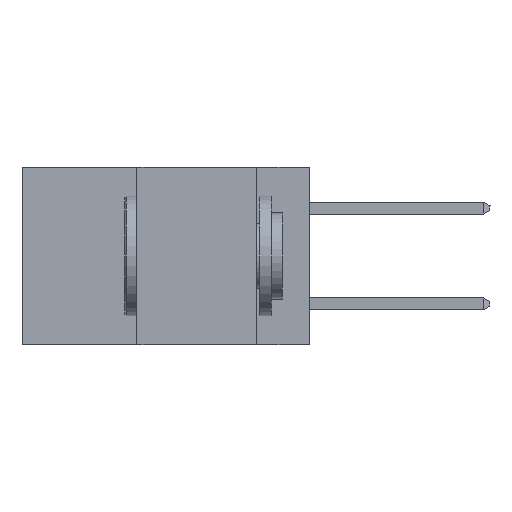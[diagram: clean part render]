
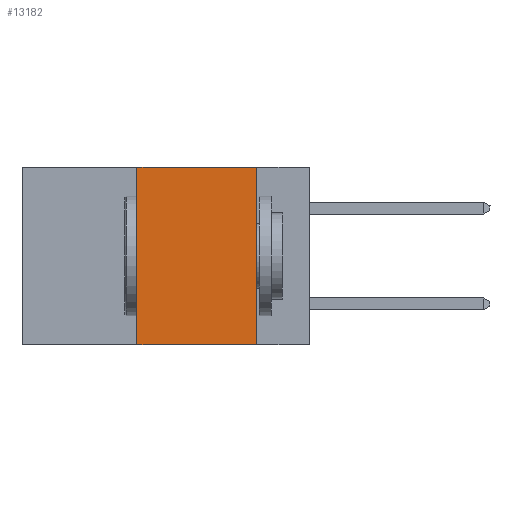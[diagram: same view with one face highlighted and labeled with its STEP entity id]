
A CAD part, left-side view. The second image highlights one B-rep face of the part: STEP entity #13182.
In plain terms, the highlighted planar face has unit normal (-1, 0, 0).
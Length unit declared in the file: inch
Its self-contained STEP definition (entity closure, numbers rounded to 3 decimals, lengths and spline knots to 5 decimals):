
#349 = ORIENTED_EDGE ( 'NONE', *, *, #10973, .F. ) ;
#589 = CARTESIAN_POINT ( 'NONE',  ( 0., 0.11, -0.37 ) ) ;
#593 = VERTEX_POINT ( 'NONE', #589 ) ;
#930 = LINE ( 'NONE', #3005, #6616 ) ;
#1371 = EDGE_CURVE ( 'NONE', #13315, #593, #5308, .T. ) ;
#1379 = CARTESIAN_POINT ( 'NONE',  ( 0., 0.6, 0. ) ) ;
#1505 = CARTESIAN_POINT ( 'NONE',  ( 0., 0.6, 0. ) ) ;
#1778 = CARTESIAN_POINT ( 'NONE',  ( 0., 0.36, -0.37 ) ) ;
#2017 = LINE ( 'NONE', #3688, #7582 ) ;
#2207 = CARTESIAN_POINT ( 'NONE',  ( 0., 0.11, 0. ) ) ;
#2328 = VECTOR ( 'NONE', #3312, 39.37008 ) ;
#2681 = DIRECTION ( 'NONE',  ( 1., 0., 0. ) ) ;
#2894 = DIRECTION ( 'NONE',  ( 0., 0., 1. ) ) ;
#3005 = CARTESIAN_POINT ( 'NONE',  ( 0., 0.36, 0. ) ) ;
#3312 = DIRECTION ( 'NONE',  ( 0., -1., 0. ) ) ;
#3688 = CARTESIAN_POINT ( 'NONE',  ( 0., 0.11, 0. ) ) ;
#3718 = FACE_OUTER_BOUND ( 'NONE', #12946, .T. ) ;
#3850 = ORIENTED_EDGE ( 'NONE', *, *, #11487, .F. ) ;
#4575 = ORIENTED_EDGE ( 'NONE', *, *, #1371, .T. ) ;
#5127 = CARTESIAN_POINT ( 'NONE',  ( 0., 0.36, 0. ) ) ;
#5267 = EDGE_CURVE ( 'NONE', #13315, #13291, #930, .T. ) ;
#5308 = LINE ( 'NONE', #5499, #2328 ) ;
#5499 = CARTESIAN_POINT ( 'NONE',  ( 0., 0.6, -0.37 ) ) ;
#5826 = AXIS2_PLACEMENT_3D ( 'NONE', #1505, #2681, #10240 ) ;
#6616 = VECTOR ( 'NONE', #2894, 39.37008 ) ;
#7582 = VECTOR ( 'NONE', #12278, 39.37008 ) ;
#8992 = LINE ( 'NONE', #1379, #11841 ) ;
#9581 = ORIENTED_EDGE ( 'NONE', *, *, #5267, .F. ) ;
#10240 = DIRECTION ( 'NONE',  ( 0., 0., -1. ) ) ;
#10747 = PLANE ( 'NONE',  #5826 ) ;
#10973 = EDGE_CURVE ( 'NONE', #11928, #593, #2017, .T. ) ;
#11200 = DIRECTION ( 'NONE',  ( 0., -1., 0. ) ) ;
#11487 = EDGE_CURVE ( 'NONE', #13291, #11928, #8992, .T. ) ;
#11841 = VECTOR ( 'NONE', #11200, 39.37008 ) ;
#11928 = VERTEX_POINT ( 'NONE', #2207 ) ;
#12278 = DIRECTION ( 'NONE',  ( 0., 0., -1. ) ) ;
#12946 = EDGE_LOOP ( 'NONE', ( #349, #3850, #9581, #4575 ) ) ;
#13182 = ADVANCED_FACE ( 'NONE', ( #3718 ), #10747, .F. ) ;
#13291 = VERTEX_POINT ( 'NONE', #5127 ) ;
#13315 = VERTEX_POINT ( 'NONE', #1778 ) ;
